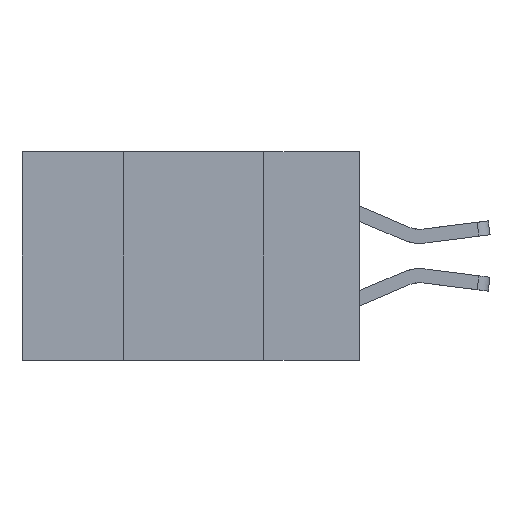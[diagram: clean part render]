
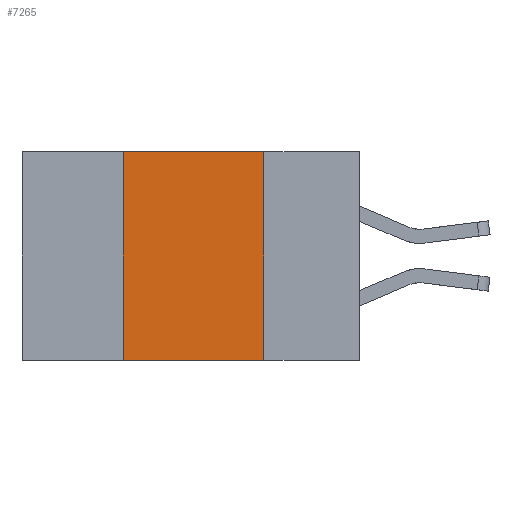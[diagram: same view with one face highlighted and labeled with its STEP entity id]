
A CAD part, left-side view. The second image highlights one B-rep face of the part: STEP entity #7265.
In plain terms, the highlighted planar face has unit normal (-1, 0, 0).
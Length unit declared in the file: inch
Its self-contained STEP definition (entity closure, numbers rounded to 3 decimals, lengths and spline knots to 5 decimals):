
#393 = LINE ( 'NONE', #4604, #6725 ) ;
#685 = VERTEX_POINT ( 'NONE', #6376 ) ;
#984 = FACE_OUTER_BOUND ( 'NONE', #6124, .T. ) ;
#1031 = VECTOR ( 'NONE', #2631, 39.37008 ) ;
#1264 = DIRECTION ( 'NONE',  ( 0., 0., 1. ) ) ;
#2631 = DIRECTION ( 'NONE',  ( 0., -1., 0. ) ) ;
#3079 = CARTESIAN_POINT ( 'NONE',  ( 0., 0.42, -0.37 ) ) ;
#3201 = VERTEX_POINT ( 'NONE', #6452 ) ;
#3370 = ORIENTED_EDGE ( 'NONE', *, *, #8582, .T. ) ;
#3397 = EDGE_CURVE ( 'NONE', #5189, #685, #9841, .T. ) ;
#3990 = DIRECTION ( 'NONE',  ( 0., 0., -1. ) ) ;
#4022 = CARTESIAN_POINT ( 'NONE',  ( 0., 0.6, 0. ) ) ;
#4072 = VERTEX_POINT ( 'NONE', #8785 ) ;
#4160 = ORIENTED_EDGE ( 'NONE', *, *, #7903, .F. ) ;
#4604 = CARTESIAN_POINT ( 'NONE',  ( 0., 0.17, 0. ) ) ;
#4957 = CARTESIAN_POINT ( 'NONE',  ( 0., 0.6, 0. ) ) ;
#5125 = LINE ( 'NONE', #4957, #1031 ) ;
#5189 = VERTEX_POINT ( 'NONE', #3079 ) ;
#6124 = EDGE_LOOP ( 'NONE', ( #8299, #4160, #8434, #3370 ) ) ;
#6307 = PLANE ( 'NONE',  #8716 ) ;
#6376 = CARTESIAN_POINT ( 'NONE',  ( 0., 0.42, 0. ) ) ;
#6452 = CARTESIAN_POINT ( 'NONE',  ( 0., 0.17, -0.37 ) ) ;
#6725 = VECTOR ( 'NONE', #7674, 39.37008 ) ;
#6755 = VECTOR ( 'NONE', #6985, 39.37008 ) ;
#6985 = DIRECTION ( 'NONE',  ( 0., -1., 0. ) ) ;
#7138 = EDGE_CURVE ( 'NONE', #4072, #3201, #393, .T. ) ;
#7265 = ADVANCED_FACE ( 'NONE', ( #984 ), #6307, .F. ) ;
#7674 = DIRECTION ( 'NONE',  ( 0., 0., -1. ) ) ;
#7688 = VECTOR ( 'NONE', #1264, 39.37008 ) ;
#7903 = EDGE_CURVE ( 'NONE', #685, #4072, #5125, .T. ) ;
#8234 = LINE ( 'NONE', #8250, #6755 ) ;
#8250 = CARTESIAN_POINT ( 'NONE',  ( 0., 0.6, -0.37 ) ) ;
#8299 = ORIENTED_EDGE ( 'NONE', *, *, #7138, .F. ) ;
#8301 = CARTESIAN_POINT ( 'NONE',  ( 0., 0.42, 0. ) ) ;
#8434 = ORIENTED_EDGE ( 'NONE', *, *, #3397, .F. ) ;
#8582 = EDGE_CURVE ( 'NONE', #5189, #3201, #8234, .T. ) ;
#8716 = AXIS2_PLACEMENT_3D ( 'NONE', #4022, #9420, #3990 ) ;
#8785 = CARTESIAN_POINT ( 'NONE',  ( 0., 0.17, 0. ) ) ;
#9420 = DIRECTION ( 'NONE',  ( 1., 0., 0. ) ) ;
#9841 = LINE ( 'NONE', #8301, #7688 ) ;
